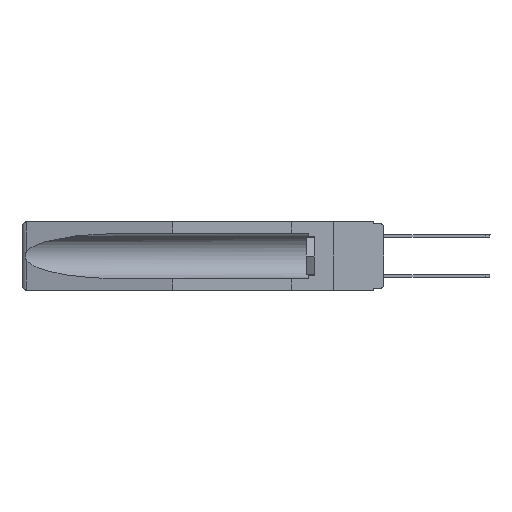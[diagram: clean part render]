
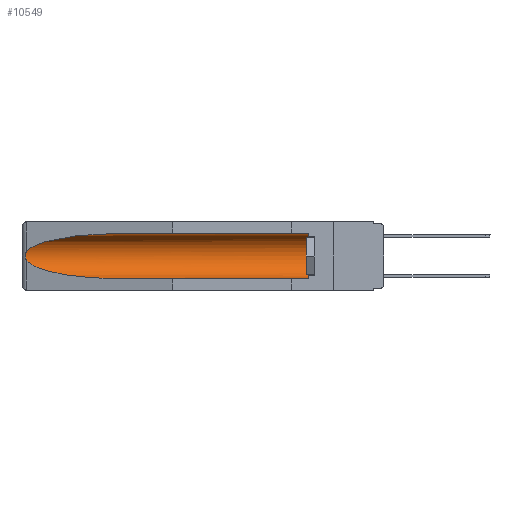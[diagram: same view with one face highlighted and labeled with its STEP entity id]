
A CAD part, left-side view. The second image highlights one B-rep face of the part: STEP entity #10549.
In plain terms, the highlighted cylindrical face has radius 2.857 mm (diameter 5.715 mm), a partial arc.
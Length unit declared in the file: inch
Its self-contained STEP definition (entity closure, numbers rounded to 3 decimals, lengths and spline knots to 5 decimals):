
#568 = CARTESIAN_POINT ( 'NONE',  ( 0.26537, 1.52718, -0.14972 ) ) ;
#690 = CARTESIAN_POINT ( 'NONE',  ( 0.26597, 1.5296, -0.19026 ) ) ;
#744 = CARTESIAN_POINT ( 'NONE',  ( 0.21114, 1.30732, -0.059 ) ) ;
#1322 = AXIS2_PLACEMENT_3D ( 'NONE', #9653, #16324, #12772 ) ;
#1696 = VECTOR ( 'NONE', #5713, 39.37008 ) ;
#1757 =( BOUNDED_CURVE ( )  B_SPLINE_CURVE ( 3, ( #9181, #11147, #19478, #12652 ),
 .UNSPECIFIED., .F., .F. ) 
 B_SPLINE_CURVE_WITH_KNOTS ( ( 4, 4 ),
 ( 0.1948, 1.5708 ),
 .UNSPECIFIED. ) 
 CURVE ( )  GEOMETRIC_REPRESENTATION_ITEM ( )  RATIONAL_B_SPLINE_CURVE ( ( 1., 0.848, 0.848, 1. ) ) 
 REPRESENTATION_ITEM ( '' )  );
#2778 = CARTESIAN_POINT ( 'NONE',  ( 0.26655, 1.53094, -0.18657 ) ) ;
#3433 = CIRCLE ( 'NONE', #16360, 0.1125 ) ;
#4114 = VERTEX_POINT ( 'NONE', #9295 ) ;
#4184 = CARTESIAN_POINT ( 'NONE',  ( 0.26654, 1.53092, -0.15636 ) ) ;
#4467 = CARTESIAN_POINT ( 'NONE',  ( 0.25451, 1.48313, -0.09465 ) ) ;
#4855 = LINE ( 'NONE', #11926, #12097 ) ;
#5224 = VERTEX_POINT ( 'NONE', #21984 ) ;
#5365 = CARTESIAN_POINT ( 'NONE',  ( 0.26537, 1.52718, -0.19328 ) ) ;
#5386 = DIRECTION ( 'NONE',  ( 0., -1., 0. ) ) ;
#5581 = EDGE_CURVE ( 'NONE', #4114, #12297, #3433, .T. ) ;
#5711 = CYLINDRICAL_SURFACE ( 'NONE', #1322, 0.1125 ) ;
#5713 = DIRECTION ( 'NONE',  ( 0., 1., 0. ) ) ;
#6059 = ORIENTED_EDGE ( 'NONE', *, *, #5581, .T. ) ;
#6156 = CARTESIAN_POINT ( 'NONE',  ( 0.2675, 1.53308, -0.16763 ) ) ;
#6185 = ORIENTED_EDGE ( 'NONE', *, *, #11932, .T. ) ;
#6315 = CARTESIAN_POINT ( 'NONE',  ( 0.26537, 1.52718, -0.14972 ) ) ;
#7331 = CARTESIAN_POINT ( 'NONE',  ( 0.155, 1.07973, -0.284 ) ) ;
#7569 = ORIENTED_EDGE ( 'NONE', *, *, #10146, .T. ) ;
#7646 = CARTESIAN_POINT ( 'NONE',  ( 0.2673, 1.5327, -0.16383 ) ) ;
#9181 = CARTESIAN_POINT ( 'NONE',  ( 0.26537, 1.52718, -0.19328 ) ) ;
#9295 = CARTESIAN_POINT ( 'NONE',  ( 0.155, 0.126, -0.284 ) ) ;
#9653 = CARTESIAN_POINT ( 'NONE',  ( 0.155, -0.30754, -0.1715 ) ) ;
#9750 = CARTESIAN_POINT ( 'NONE',  ( 0.26597, 1.52961, -0.15275 ) ) ;
#10146 = EDGE_CURVE ( 'NONE', #5224, #22697, #18353, .T. ) ;
#10234 = CARTESIAN_POINT ( 'NONE',  ( 0.155, 0.126, -0.059 ) ) ;
#10549 = ADVANCED_FACE ( 'NONE', ( #21584 ), #5711, .F. ) ;
#10597 = CARTESIAN_POINT ( 'NONE',  ( 0.155, -0.30754, -0.059 ) ) ;
#11065 = CARTESIAN_POINT ( 'NONE',  ( 0.155, 1.07973, -0.059 ) ) ;
#11147 = CARTESIAN_POINT ( 'NONE',  ( 0.25451, 1.48313, -0.24835 ) ) ;
#11775 = ORIENTED_EDGE ( 'NONE', *, *, #17109, .T. ) ;
#11926 = CARTESIAN_POINT ( 'NONE',  ( 0.155, -0.30754, -0.284 ) ) ;
#11932 = EDGE_CURVE ( 'NONE', #12297, #5224, #14050, .T. ) ;
#12097 = VECTOR ( 'NONE', #18982, 39.37008 ) ;
#12297 = VERTEX_POINT ( 'NONE', #10234 ) ;
#12652 = CARTESIAN_POINT ( 'NONE',  ( 0.155, 1.07973, -0.284 ) ) ;
#12772 = DIRECTION ( 'NONE',  ( 0., 0., 1. ) ) ;
#12839 = EDGE_CURVE ( 'NONE', #4114, #19436, #4855, .T. ) ;
#13108 = CARTESIAN_POINT ( 'NONE',  ( 0.2673, 1.53269, -0.17917 ) ) ;
#13339 = CARTESIAN_POINT ( 'NONE',  ( 0.2675, 1.53308, -0.17534 ) ) ;
#14050 = LINE ( 'NONE', #10597, #1696 ) ;
#14068 = CARTESIAN_POINT ( 'NONE',  ( 0.155, 0.126, -0.1715 ) ) ;
#14290 = DIRECTION ( 'NONE',  ( 0., 0., 1. ) ) ;
#14704 = CARTESIAN_POINT ( 'NONE',  ( 0.26537, 1.52718, -0.19328 ) ) ;
#15645 = ORIENTED_EDGE ( 'NONE', *, *, #21371, .T. ) ;
#16324 = DIRECTION ( 'NONE',  ( 0., 1., 0. ) ) ;
#16360 = AXIS2_PLACEMENT_3D ( 'NONE', #14068, #5386, #14290 ) ;
#16469 = EDGE_LOOP ( 'NONE', ( #7569, #11775, #15645, #16904, #6059, #6185 ) ) ;
#16904 = ORIENTED_EDGE ( 'NONE', *, *, #12839, .F. ) ;
#17041 = B_SPLINE_CURVE_WITH_KNOTS ( 'NONE', 3,
 ( #568, #9750, #4184, #7646, #6156, #13339, #13108, #2778, #690, #14704 ),
 .UNSPECIFIED., .F., .F.,
 ( 4, 2, 2, 2, 4 ),
 ( 0., 0.00029, 0.00058, 0.00087, 0.00117 ),
 .UNSPECIFIED. ) ;
#17109 = EDGE_CURVE ( 'NONE', #22697, #22578, #17041, .T. ) ;
#18353 =( BOUNDED_CURVE ( )  B_SPLINE_CURVE ( 3, ( #11065, #744, #4467, #6315 ),
 .UNSPECIFIED., .F., .F. ) 
 B_SPLINE_CURVE_WITH_KNOTS ( ( 4, 4 ),
 ( 4.71239, 6.08839 ),
 .UNSPECIFIED. ) 
 CURVE ( )  GEOMETRIC_REPRESENTATION_ITEM ( )  RATIONAL_B_SPLINE_CURVE ( ( 1., 0.848, 0.848, 1. ) ) 
 REPRESENTATION_ITEM ( '' )  );
#18982 = DIRECTION ( 'NONE',  ( 0., 1., 0. ) ) ;
#19436 = VERTEX_POINT ( 'NONE', #7331 ) ;
#19478 = CARTESIAN_POINT ( 'NONE',  ( 0.21114, 1.30732, -0.284 ) ) ;
#21371 = EDGE_CURVE ( 'NONE', #22578, #19436, #1757, .T. ) ;
#21584 = FACE_OUTER_BOUND ( 'NONE', #16469, .T. ) ;
#21818 = CARTESIAN_POINT ( 'NONE',  ( 0.26537, 1.52718, -0.14972 ) ) ;
#21984 = CARTESIAN_POINT ( 'NONE',  ( 0.155, 1.07973, -0.059 ) ) ;
#22578 = VERTEX_POINT ( 'NONE', #5365 ) ;
#22697 = VERTEX_POINT ( 'NONE', #21818 ) ;
